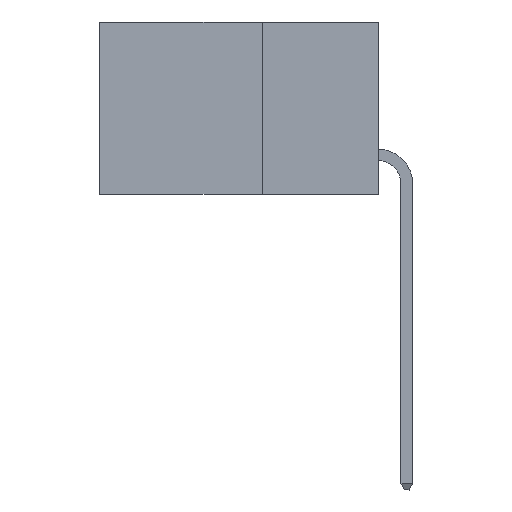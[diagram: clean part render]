
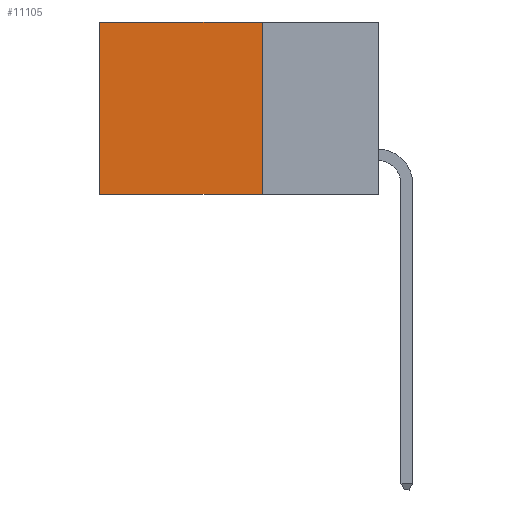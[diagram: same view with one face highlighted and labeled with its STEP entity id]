
A CAD part, left-side view. The second image highlights one B-rep face of the part: STEP entity #11105.
In plain terms, the highlighted planar face has unit normal (-1, 0, 0).
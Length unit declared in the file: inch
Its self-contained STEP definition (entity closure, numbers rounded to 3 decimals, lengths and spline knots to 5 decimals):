
#739 = DIRECTION ( 'NONE',  ( 0., 0., -1. ) ) ;
#1302 = VERTEX_POINT ( 'NONE', #6085 ) ;
#2481 = VERTEX_POINT ( 'NONE', #8402 ) ;
#3047 = VECTOR ( 'NONE', #16510, 39.37008 ) ;
#3976 = PLANE ( 'NONE',  #5979 ) ;
#4063 = CARTESIAN_POINT ( 'NONE',  ( 0.298, 0.25, 0. ) ) ;
#5353 = FACE_OUTER_BOUND ( 'NONE', #7658, .T. ) ;
#5519 = EDGE_CURVE ( 'NONE', #16405, #1302, #6720, .T. ) ;
#5979 = AXIS2_PLACEMENT_3D ( 'NONE', #13314, #14540, #6742 ) ;
#6085 = CARTESIAN_POINT ( 'NONE',  ( 0.298, 0.6, -0.37 ) ) ;
#6693 = LINE ( 'NONE', #8857, #3047 ) ;
#6720 = LINE ( 'NONE', #15190, #13316 ) ;
#6742 = DIRECTION ( 'NONE',  ( 0., 0., -1. ) ) ;
#7604 = CARTESIAN_POINT ( 'NONE',  ( 0.298, 0.25, 0. ) ) ;
#7658 = EDGE_LOOP ( 'NONE', ( #13758, #14242, #13672, #8266 ) ) ;
#7802 = CARTESIAN_POINT ( 'NONE',  ( 0.298, 0.25, -0.37 ) ) ;
#8266 = ORIENTED_EDGE ( 'NONE', *, *, #12213, .T. ) ;
#8402 = CARTESIAN_POINT ( 'NONE',  ( 0.298, 0.6, 0. ) ) ;
#8537 = VERTEX_POINT ( 'NONE', #4063 ) ;
#8857 = CARTESIAN_POINT ( 'NONE',  ( 0.298, 0.6, 0. ) ) ;
#9295 = EDGE_CURVE ( 'NONE', #8537, #16405, #16824, .T. ) ;
#9769 = DIRECTION ( 'NONE',  ( 0., 1., 0. ) ) ;
#10474 = VECTOR ( 'NONE', #739, 39.37008 ) ;
#10983 = VECTOR ( 'NONE', #9769, 39.37008 ) ;
#11105 = ADVANCED_FACE ( 'NONE', ( #5353 ), #3976, .F. ) ;
#12213 = EDGE_CURVE ( 'NONE', #8537, #2481, #14372, .T. ) ;
#13314 = CARTESIAN_POINT ( 'NONE',  ( 0.298, 0.25, 0. ) ) ;
#13316 = VECTOR ( 'NONE', #16517, 39.37008 ) ;
#13576 = CARTESIAN_POINT ( 'NONE',  ( 0.298, 0.25, 0. ) ) ;
#13672 = ORIENTED_EDGE ( 'NONE', *, *, #9295, .F. ) ;
#13758 = ORIENTED_EDGE ( 'NONE', *, *, #15764, .T. ) ;
#14242 = ORIENTED_EDGE ( 'NONE', *, *, #5519, .F. ) ;
#14372 = LINE ( 'NONE', #13576, #10983 ) ;
#14540 = DIRECTION ( 'NONE',  ( 1., 0., 0. ) ) ;
#15190 = CARTESIAN_POINT ( 'NONE',  ( 0.298, 0.25, -0.37 ) ) ;
#15764 = EDGE_CURVE ( 'NONE', #2481, #1302, #6693, .T. ) ;
#16405 = VERTEX_POINT ( 'NONE', #7802 ) ;
#16510 = DIRECTION ( 'NONE',  ( 0., 0., -1. ) ) ;
#16517 = DIRECTION ( 'NONE',  ( 0., 1., 0. ) ) ;
#16824 = LINE ( 'NONE', #7604, #10474 ) ;
